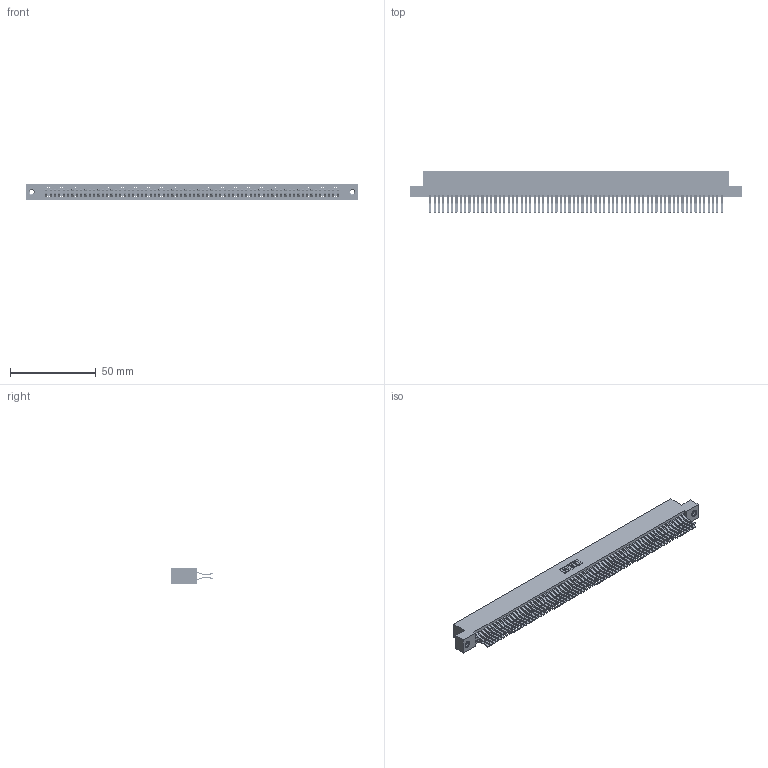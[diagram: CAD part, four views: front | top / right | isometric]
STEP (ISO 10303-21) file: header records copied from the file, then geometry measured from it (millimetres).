
FILE_DESCRIPTION (( 'STEP AP203' ), '1' );
FILE_NAME ('345-136-560-208.STEP', '2019-11-08T12:00:13', ( '' ), ( '' ), 'SwSTEP 2.0', 'SolidWorks 2016', '' );
FILE_SCHEMA (( 'CONFIG_CONTROL_DESIGN' ));
Length unit declared in the file: inch
Products named in the file (4): 345-136-560-208; 345-292-001_560 Tail; 345 Part_Flush Mounting Lugs - 0.156 Dia-TI; 345-250-001_345-250-003-102
Assembly tree (139 placements, depth 2):
  345-136-560-208
    345 Part_Flush Mounting Lugs - 0.156 Dia-TI
    345-292-001_560 Tail  x136
    345-250-001_345-250-003-102  x2
Bounding box: 193.93 x 24.45 x 9.4 mm (x, y, z)
Volume: 19964.7 mm3; surface area: 32320.8 mm2
Topology: 139 solids, 139 shells, 7258 faces, 21557 edges, 14182 vertices
Faces by surface type: plane 4600, cylinder 2642, cone 12, torus 4
Entity records: 51128 total; most frequent: CARTESIAN_POINT 8527, ORIENTED_EDGE 8454, DIRECTION 7517, EDGE_CURVE 4227, VECTOR 3799, LINE 3799, VERTEX_POINT 2812, AXIS2_PLACEMENT_3D 1859
